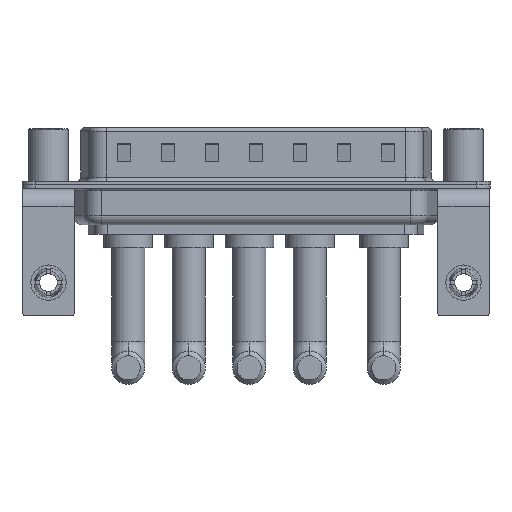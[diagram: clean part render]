
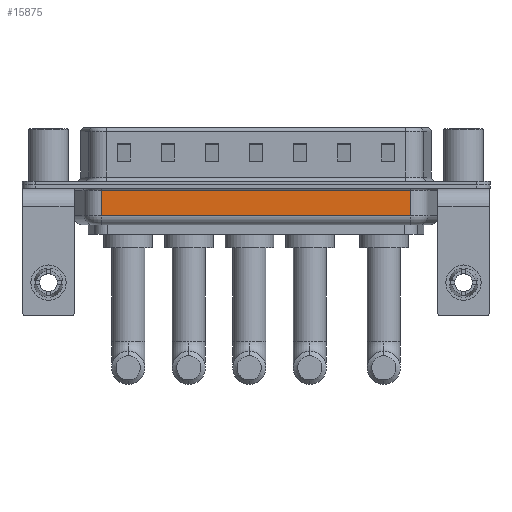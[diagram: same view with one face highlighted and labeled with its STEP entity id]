
A CAD part, front view. The second image highlights one B-rep face of the part: STEP entity #15875.
In plain terms, the highlighted planar face has unit normal (0, -1, 0).
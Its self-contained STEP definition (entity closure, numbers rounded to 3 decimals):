
#1024 = VERTEX_POINT ( 'NONE', #7228 ) ;
#1726 = EDGE_CURVE ( 'NONE', #12774, #11099, #12137, .T. ) ;
#1856 = ORIENTED_EDGE ( 'NONE', *, *, #1726, .T. ) ;
#2538 = EDGE_CURVE ( 'NONE', #11099, #1024, #14984, .T. ) ;
#2574 = CARTESIAN_POINT ( 'NONE',  ( 6.006, -5.35, -0.65 ) ) ;
#3823 = VECTOR ( 'NONE', #8082, 1000. ) ;
#4171 = LINE ( 'NONE', #9697, #13347 ) ;
#4264 = CARTESIAN_POINT ( 'NONE',  ( 41.044, -5.35, -4.5 ) ) ;
#5001 = CARTESIAN_POINT ( 'NONE',  ( 41.044, -5.35, -0.65 ) ) ;
#5160 = PLANE ( 'NONE',  #5645 ) ;
#5472 = CARTESIAN_POINT ( 'NONE',  ( 41.044, -5.35, -3.5 ) ) ;
#5481 = ORIENTED_EDGE ( 'NONE', *, *, #2538, .T. ) ;
#5586 = CARTESIAN_POINT ( 'NONE',  ( 6.006, -5.35, -4.5 ) ) ;
#5645 = AXIS2_PLACEMENT_3D ( 'NONE', #6523, #9154, #7869 ) ;
#5852 = LINE ( 'NONE', #5586, #15955 ) ;
#6523 = CARTESIAN_POINT ( 'NONE',  ( 6.006, -5.35, -4.5 ) ) ;
#7228 = CARTESIAN_POINT ( 'NONE',  ( 6.006, -5.35, -0.65 ) ) ;
#7869 = DIRECTION ( 'NONE',  ( 0., 0., 1. ) ) ;
#8082 = DIRECTION ( 'NONE',  ( -1., 0., 0. ) ) ;
#8377 = EDGE_LOOP ( 'NONE', ( #13970, #12847, #1856, #5481 ) ) ;
#9154 = DIRECTION ( 'NONE',  ( 0., 1., 0. ) ) ;
#9697 = CARTESIAN_POINT ( 'NONE',  ( 6.006, -5.35, -3.5 ) ) ;
#9843 = CARTESIAN_POINT ( 'NONE',  ( 6.006, -5.35, -3.5 ) ) ;
#11099 = VERTEX_POINT ( 'NONE', #5001 ) ;
#11380 = DIRECTION ( 'NONE',  ( 0., 0., 1. ) ) ;
#11676 = VERTEX_POINT ( 'NONE', #9843 ) ;
#11728 = EDGE_CURVE ( 'NONE', #11676, #1024, #5852, .T. ) ;
#12137 = LINE ( 'NONE', #4264, #16534 ) ;
#12226 = EDGE_CURVE ( 'NONE', #11676, #12774, #4171, .T. ) ;
#12492 = DIRECTION ( 'NONE',  ( 0., 0., 1. ) ) ;
#12774 = VERTEX_POINT ( 'NONE', #5472 ) ;
#12847 = ORIENTED_EDGE ( 'NONE', *, *, #12226, .T. ) ;
#13347 = VECTOR ( 'NONE', #15220, 1000. ) ;
#13970 = ORIENTED_EDGE ( 'NONE', *, *, #11728, .F. ) ;
#14984 = LINE ( 'NONE', #2574, #3823 ) ;
#15220 = DIRECTION ( 'NONE',  ( 1., 0., 0. ) ) ;
#15875 = ADVANCED_FACE ( 'NONE', ( #17590 ), #5160, .F. ) ;
#15955 = VECTOR ( 'NONE', #11380, 1000. ) ;
#16534 = VECTOR ( 'NONE', #12492, 1000. ) ;
#17590 = FACE_OUTER_BOUND ( 'NONE', #8377, .T. ) ;
